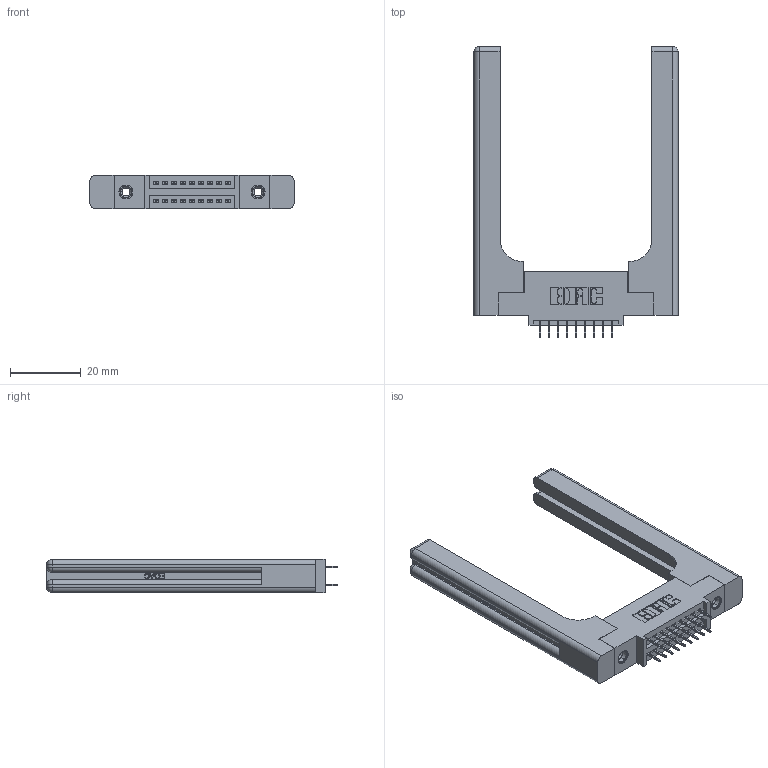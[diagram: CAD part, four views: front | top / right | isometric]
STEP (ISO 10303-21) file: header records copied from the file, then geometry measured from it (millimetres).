
FILE_DESCRIPTION (( 'STEP AP203' ), '1' );
FILE_NAME ('395-018-525-558.STEP', '2020-09-23T11:04:19', ( '' ), ( '' ), 'SwSTEP 2.0', 'SolidWorks 2020', '' );
FILE_SCHEMA (( 'CONFIG_CONTROL_DESIGN' ));
Length unit declared in the file: inch
Products named in the file (5): 345 Part_0.110 Offset - 0.156 Dia-TH; 345-250-001_345-250-001-102; 345-292-001_345-293-125; 345-220-058_345-220-058; 395-018-525-558
Assembly tree (23 placements, depth 2):
  395-018-525-558
    345 Part_0.110 Offset - 0.156 Dia-TH
    345-292-001_345-293-125  x18
    345-250-001_345-250-001-102  x2
    345-220-058_345-220-058  x2
Bounding box: 57.89 x 82.47 x 9.4 mm (x, y, z)
Volume: 13689 mm3; surface area: 12130.2 mm2
Topology: 23 solids, 23 shells, 1358 faces, 3773 edges, 2422 vertices
Faces by surface type: plane 934, cylinder 364, bspline 36, cone 12, sphere 8, torus 4
Entity records: 16892 total; most frequent: CARTESIAN_POINT 3857, ORIENTED_EDGE 2588, DIRECTION 2374, EDGE_CURVE 1294, LINE 1038, VECTOR 1038, VERTEX_POINT 850, AXIS2_PLACEMENT_3D 668
